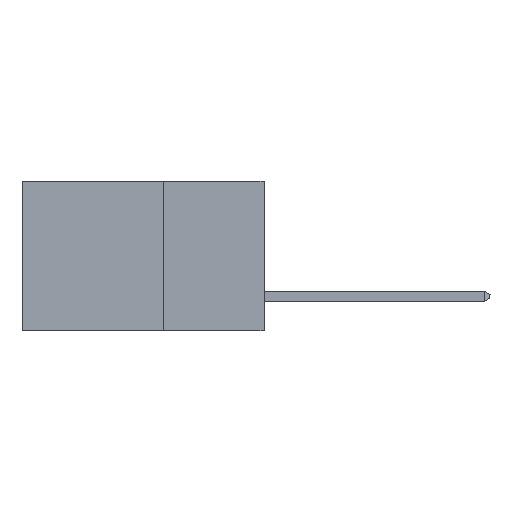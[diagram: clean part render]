
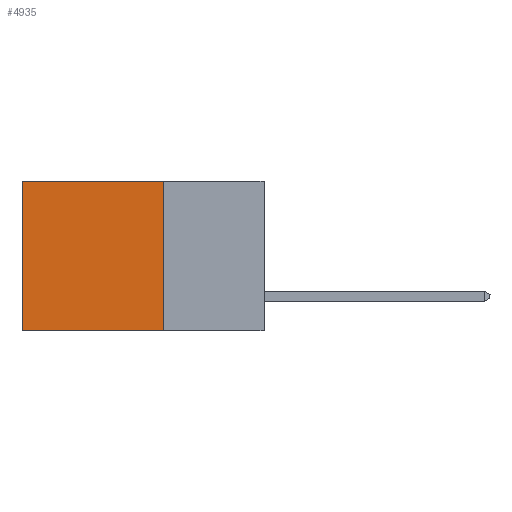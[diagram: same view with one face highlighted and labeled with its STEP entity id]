
A CAD part, left-side view. The second image highlights one B-rep face of the part: STEP entity #4935.
In plain terms, the highlighted planar face has unit normal (-1, 0, 0).
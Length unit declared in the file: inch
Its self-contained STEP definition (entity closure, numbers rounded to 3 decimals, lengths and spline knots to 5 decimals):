
#18 = VERTEX_POINT ( 'NONE', #13802 ) ;
#212 = DIRECTION ( 'NONE',  ( 0., 0., -1. ) ) ;
#674 = LINE ( 'NONE', #2079, #12785 ) ;
#2079 = CARTESIAN_POINT ( 'NONE',  ( 0.2615, 0.25, -0.37 ) ) ;
#2629 = LINE ( 'NONE', #9963, #14114 ) ;
#3902 = ORIENTED_EDGE ( 'NONE', *, *, #11655, .T. ) ;
#4896 = LINE ( 'NONE', #6189, #14237 ) ;
#4935 = ADVANCED_FACE ( 'NONE', ( #11696 ), #12775, .F. ) ;
#5362 = VERTEX_POINT ( 'NONE', #11978 ) ;
#5805 = CARTESIAN_POINT ( 'NONE',  ( 0.2615, 0.25, -0.37 ) ) ;
#6189 = CARTESIAN_POINT ( 'NONE',  ( 0.2615, 0.25, 0. ) ) ;
#6388 = DIRECTION ( 'NONE',  ( 0., 1., 0. ) ) ;
#6969 = AXIS2_PLACEMENT_3D ( 'NONE', #5805, #7038, #11631 ) ;
#7038 = DIRECTION ( 'NONE',  ( 1., 0., 0. ) ) ;
#7441 = DIRECTION ( 'NONE',  ( 0., 1., 0. ) ) ;
#9152 = VERTEX_POINT ( 'NONE', #12398 ) ;
#9304 = VECTOR ( 'NONE', #212, 39.37008 ) ;
#9899 = EDGE_CURVE ( 'NONE', #18, #5362, #4896, .T. ) ;
#9963 = CARTESIAN_POINT ( 'NONE',  ( 0.2615, 0.25, -0.37 ) ) ;
#10071 = EDGE_CURVE ( 'NONE', #18, #9152, #674, .T. ) ;
#10138 = DIRECTION ( 'NONE',  ( 0., 0., -1. ) ) ;
#10830 = CARTESIAN_POINT ( 'NONE',  ( 0.2615, 0.6, -0.37 ) ) ;
#11146 = ORIENTED_EDGE ( 'NONE', *, *, #10071, .F. ) ;
#11631 = DIRECTION ( 'NONE',  ( 0., 0., -1. ) ) ;
#11655 = EDGE_CURVE ( 'NONE', #5362, #12767, #11993, .T. ) ;
#11696 = FACE_OUTER_BOUND ( 'NONE', #13287, .T. ) ;
#11978 = CARTESIAN_POINT ( 'NONE',  ( 0.2615, 0.6, 0. ) ) ;
#11993 = LINE ( 'NONE', #10830, #9304 ) ;
#12398 = CARTESIAN_POINT ( 'NONE',  ( 0.2615, 0.25, -0.37 ) ) ;
#12767 = VERTEX_POINT ( 'NONE', #13938 ) ;
#12775 = PLANE ( 'NONE',  #6969 ) ;
#12785 = VECTOR ( 'NONE', #10138, 39.37008 ) ;
#13262 = ORIENTED_EDGE ( 'NONE', *, *, #14283, .F. ) ;
#13287 = EDGE_LOOP ( 'NONE', ( #3902, #13262, #11146, #13509 ) ) ;
#13509 = ORIENTED_EDGE ( 'NONE', *, *, #9899, .T. ) ;
#13802 = CARTESIAN_POINT ( 'NONE',  ( 0.2615, 0.25, 0. ) ) ;
#13938 = CARTESIAN_POINT ( 'NONE',  ( 0.2615, 0.6, -0.37 ) ) ;
#14114 = VECTOR ( 'NONE', #6388, 39.37008 ) ;
#14237 = VECTOR ( 'NONE', #7441, 39.37008 ) ;
#14283 = EDGE_CURVE ( 'NONE', #9152, #12767, #2629, .T. ) ;
